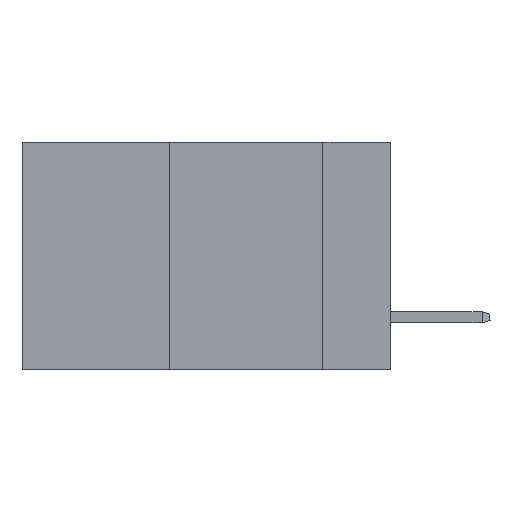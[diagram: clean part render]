
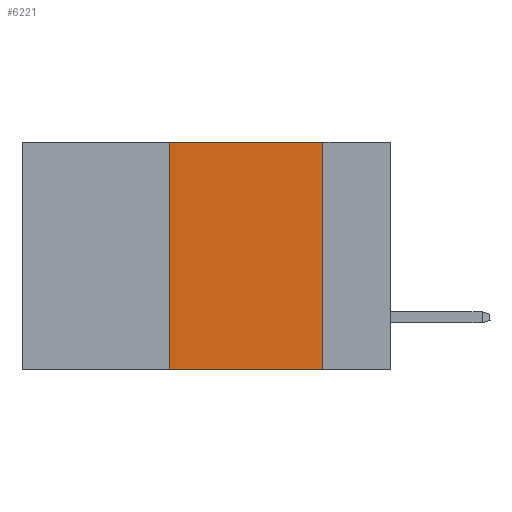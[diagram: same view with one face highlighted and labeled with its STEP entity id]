
A CAD part, left-side view. The second image highlights one B-rep face of the part: STEP entity #6221.
In plain terms, the highlighted planar face has unit normal (-1, 0, 0).
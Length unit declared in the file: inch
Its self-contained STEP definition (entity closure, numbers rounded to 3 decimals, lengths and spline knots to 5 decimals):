
#178 = CARTESIAN_POINT ( 'NONE',  ( 0., 0.6, 0. ) ) ;
#329 = PLANE ( 'NONE',  #18852 ) ;
#388 = VECTOR ( 'NONE', #19000, 39.37008 ) ;
#691 = EDGE_CURVE ( 'NONE', #5875, #30942, #8432, .T. ) ;
#912 = CARTESIAN_POINT ( 'NONE',  ( 0., 0.11, 0. ) ) ;
#1555 = LINE ( 'NONE', #30745, #388 ) ;
#4844 = DIRECTION ( 'NONE',  ( 0., 0., 1. ) ) ;
#5130 = CARTESIAN_POINT ( 'NONE',  ( 0., 0.36, -0.37 ) ) ;
#5515 = ORIENTED_EDGE ( 'NONE', *, *, #19245, .T. ) ;
#5553 = DIRECTION ( 'NONE',  ( 1., 0., 0. ) ) ;
#5875 = VERTEX_POINT ( 'NONE', #13562 ) ;
#6221 = ADVANCED_FACE ( 'NONE', ( #20541 ), #329, .F. ) ;
#6628 = EDGE_LOOP ( 'NONE', ( #24848, #13412, #30530, #5515 ) ) ;
#7612 = CARTESIAN_POINT ( 'NONE',  ( 0., 0.36, 0. ) ) ;
#8432 = LINE ( 'NONE', #912, #23915 ) ;
#11217 = LINE ( 'NONE', #17892, #18628 ) ;
#12931 = VECTOR ( 'NONE', #4844, 39.37008 ) ;
#13412 = ORIENTED_EDGE ( 'NONE', *, *, #29903, .F. ) ;
#13562 = CARTESIAN_POINT ( 'NONE',  ( 0., 0.11, 0. ) ) ;
#15492 = DIRECTION ( 'NONE',  ( 0., 0., -1. ) ) ;
#17171 = VERTEX_POINT ( 'NONE', #5130 ) ;
#17377 = LINE ( 'NONE', #7612, #12931 ) ;
#17892 = CARTESIAN_POINT ( 'NONE',  ( 0., 0.6, 0. ) ) ;
#18628 = VECTOR ( 'NONE', #30444, 39.37008 ) ;
#18852 = AXIS2_PLACEMENT_3D ( 'NONE', #178, #5553, #15492 ) ;
#19000 = DIRECTION ( 'NONE',  ( 0., -1., 0. ) ) ;
#19245 = EDGE_CURVE ( 'NONE', #17171, #30942, #1555, .T. ) ;
#20541 = FACE_OUTER_BOUND ( 'NONE', #6628, .T. ) ;
#20804 = DIRECTION ( 'NONE',  ( 0., 0., -1. ) ) ;
#21835 = VERTEX_POINT ( 'NONE', #28687 ) ;
#23915 = VECTOR ( 'NONE', #20804, 39.37008 ) ;
#24848 = ORIENTED_EDGE ( 'NONE', *, *, #691, .F. ) ;
#27344 = CARTESIAN_POINT ( 'NONE',  ( 0., 0.11, -0.37 ) ) ;
#28687 = CARTESIAN_POINT ( 'NONE',  ( 0., 0.36, 0. ) ) ;
#29903 = EDGE_CURVE ( 'NONE', #21835, #5875, #11217, .T. ) ;
#30206 = EDGE_CURVE ( 'NONE', #17171, #21835, #17377, .T. ) ;
#30444 = DIRECTION ( 'NONE',  ( 0., -1., 0. ) ) ;
#30530 = ORIENTED_EDGE ( 'NONE', *, *, #30206, .F. ) ;
#30745 = CARTESIAN_POINT ( 'NONE',  ( 0., 0.6, -0.37 ) ) ;
#30942 = VERTEX_POINT ( 'NONE', #27344 ) ;
